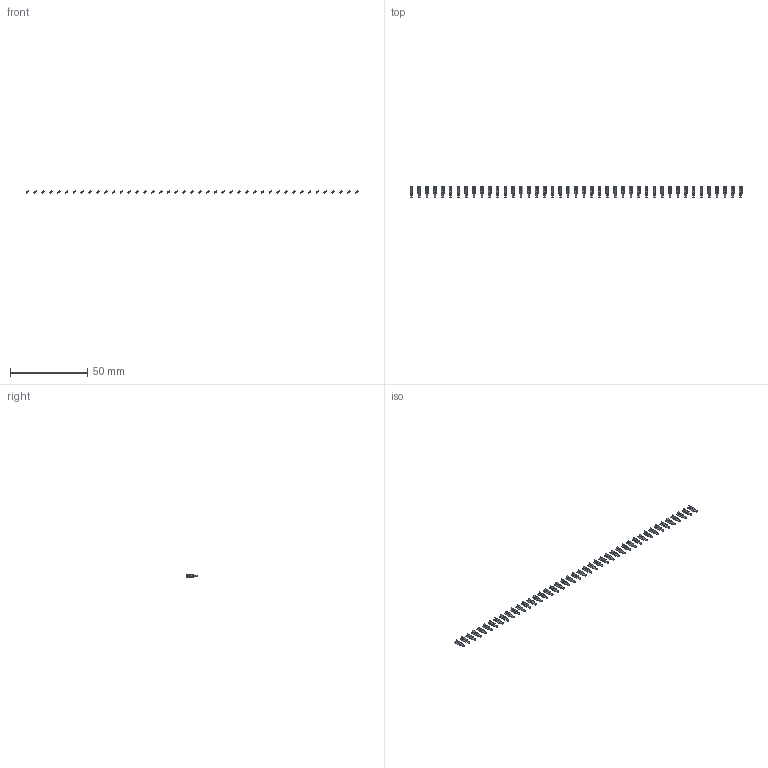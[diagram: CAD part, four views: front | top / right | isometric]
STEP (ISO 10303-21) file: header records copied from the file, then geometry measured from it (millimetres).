
FILE_DESCRIPTION (( 'STEP AP203' ), '1' );
FILE_NAME ('106-043-253-200.STEP', '2020-04-16T20:20:23', ( '' ), ( '' ), 'SwSTEP 2.0', 'SolidWorks 2016', '' );
FILE_SCHEMA (( 'CONFIG_CONTROL_DESIGN' ));
Length unit declared in the file: inch
Products named in the file (2): 100-290-001_100-290-253; 106-043-253-200
Assembly tree (43 placements, depth 2):
  106-043-253-200
    100-290-001_100-290-253  x43
Bounding box: 215.16 x 7.62 x 1.8 mm (x, y, z)
Volume: 237.3 mm3; surface area: 1479.5 mm2
Topology: 43 solids, 43 shells, 860 faces, 2322 edges, 1548 vertices
Faces by surface type: plane 817, cylinder 43
Entity records: 2164 total; most frequent: DIRECTION 188, CARTESIAN_POINT 156, ORIENTED_EDGE 108, COORDINATED_UNIVERSAL_TIME_OFFSET 96, CALENDAR_DATE 96, LOCAL_TIME 96, DATE_AND_TIME 96, AXIS2_PLACEMENT_3D 68
